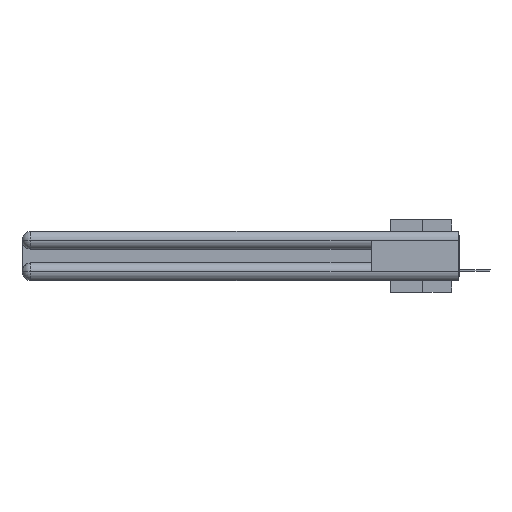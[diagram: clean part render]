
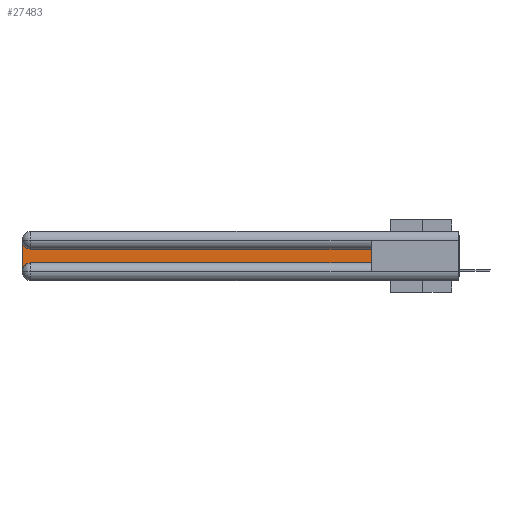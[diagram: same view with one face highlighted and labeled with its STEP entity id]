
A CAD part, left-side view. The second image highlights one B-rep face of the part: STEP entity #27483.
In plain terms, the highlighted planar face has unit normal (-1, 0, 0).
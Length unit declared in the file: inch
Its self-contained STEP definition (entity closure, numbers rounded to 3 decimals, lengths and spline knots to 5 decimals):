
#432 = ORIENTED_EDGE ( 'NONE', *, *, #32829, .T. ) ;
#638 = CARTESIAN_POINT ( 'NONE',  ( 0.075, 2.94, -0.1225 ) ) ;
#1663 = CARTESIAN_POINT ( 'NONE',  ( 0.075, 2.94, -0.0625 ) ) ;
#1751 = LINE ( 'NONE', #15003, #8052 ) ;
#2339 = DIRECTION ( 'NONE',  ( 0., 0., -1. ) ) ;
#2362 = DIRECTION ( 'NONE',  ( 0., 0., -1. ) ) ;
#3739 = LINE ( 'NONE', #13829, #25757 ) ;
#4275 = ORIENTED_EDGE ( 'NONE', *, *, #29544, .T. ) ;
#5018 = DIRECTION ( 'NONE',  ( 1., 0., 0. ) ) ;
#5976 = AXIS2_PLACEMENT_3D ( 'NONE', #21075, #18773, #2339 ) ;
#6886 = DIRECTION ( 'NONE',  ( 0., 1., 0. ) ) ;
#7191 = EDGE_CURVE ( 'NONE', #20240, #17001, #10913, .T. ) ;
#8052 = VECTOR ( 'NONE', #6886, 39.37008 ) ;
#8986 = CARTESIAN_POINT ( 'NONE',  ( 0.075, 2.94, -0.2175 ) ) ;
#9377 = CARTESIAN_POINT ( 'NONE',  ( 0.075, 3., -0.2775 ) ) ;
#9641 = VERTEX_POINT ( 'NONE', #12288 ) ;
#10397 = DIRECTION ( 'NONE',  ( 0., 0., -1. ) ) ;
#10913 = CIRCLE ( 'NONE', #23324, 0.06 ) ;
#11377 = VERTEX_POINT ( 'NONE', #8986 ) ;
#12288 = CARTESIAN_POINT ( 'NONE',  ( 0.075, 0.6, -0.1225 ) ) ;
#12927 = ORIENTED_EDGE ( 'NONE', *, *, #19563, .T. ) ;
#13038 = LINE ( 'NONE', #18873, #29145 ) ;
#13288 = FACE_OUTER_BOUND ( 'NONE', #18052, .T. ) ;
#13829 = CARTESIAN_POINT ( 'NONE',  ( 0.075, 0.6, -0.2175 ) ) ;
#13976 = ORIENTED_EDGE ( 'NONE', *, *, #27646, .T. ) ;
#14682 = VECTOR ( 'NONE', #24218, 39.37008 ) ;
#15003 = CARTESIAN_POINT ( 'NONE',  ( 0.075, 0.6, -0.1225 ) ) ;
#15556 = CARTESIAN_POINT ( 'NONE',  ( 0.075, 0.6, -0.2175 ) ) ;
#16238 = LINE ( 'NONE', #32523, #14682 ) ;
#17001 = VERTEX_POINT ( 'NONE', #26460 ) ;
#17504 = ORIENTED_EDGE ( 'NONE', *, *, #24723, .T. ) ;
#18052 = EDGE_LOOP ( 'NONE', ( #17504, #34514, #4275, #12927, #432, #13976 ) ) ;
#18773 = DIRECTION ( 'NONE',  ( 1., 0., 0. ) ) ;
#18873 = CARTESIAN_POINT ( 'NONE',  ( 0.075, 3., -0.2175 ) ) ;
#19563 = EDGE_CURVE ( 'NONE', #26129, #11377, #21704, .T. ) ;
#20240 = VERTEX_POINT ( 'NONE', #638 ) ;
#21075 = CARTESIAN_POINT ( 'NONE',  ( 0.075, 3., -0.1225 ) ) ;
#21704 = CIRCLE ( 'NONE', #31845, 0.06 ) ;
#23324 = AXIS2_PLACEMENT_3D ( 'NONE', #1663, #5018, #2362 ) ;
#24218 = DIRECTION ( 'NONE',  ( 0., -1., 0. ) ) ;
#24723 = EDGE_CURVE ( 'NONE', #9641, #20240, #1751, .T. ) ;
#25757 = VECTOR ( 'NONE', #32742, 39.37008 ) ;
#26129 = VERTEX_POINT ( 'NONE', #9377 ) ;
#26460 = CARTESIAN_POINT ( 'NONE',  ( 0.075, 3., -0.0625 ) ) ;
#27483 = ADVANCED_FACE ( 'NONE', ( #13288 ), #29210, .F. ) ;
#27646 = EDGE_CURVE ( 'NONE', #33963, #9641, #3739, .T. ) ;
#28632 = CARTESIAN_POINT ( 'NONE',  ( 0.075, 2.94, -0.2775 ) ) ;
#28811 = DIRECTION ( 'NONE',  ( 1., 0., 0. ) ) ;
#29145 = VECTOR ( 'NONE', #10397, 39.37008 ) ;
#29210 = PLANE ( 'NONE',  #5976 ) ;
#29544 = EDGE_CURVE ( 'NONE', #17001, #26129, #13038, .T. ) ;
#31845 = AXIS2_PLACEMENT_3D ( 'NONE', #28632, #28811, #33765 ) ;
#32523 = CARTESIAN_POINT ( 'NONE',  ( 0.075, 0.6, -0.2175 ) ) ;
#32742 = DIRECTION ( 'NONE',  ( 0., 0., 1. ) ) ;
#32829 = EDGE_CURVE ( 'NONE', #11377, #33963, #16238, .T. ) ;
#33765 = DIRECTION ( 'NONE',  ( 0., 0., -1. ) ) ;
#33963 = VERTEX_POINT ( 'NONE', #15556 ) ;
#34514 = ORIENTED_EDGE ( 'NONE', *, *, #7191, .T. ) ;
